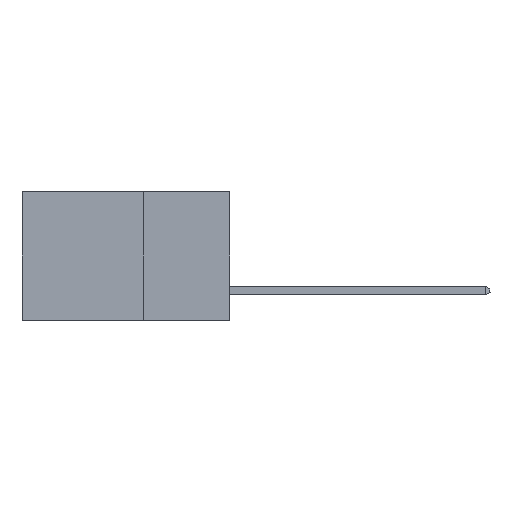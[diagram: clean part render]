
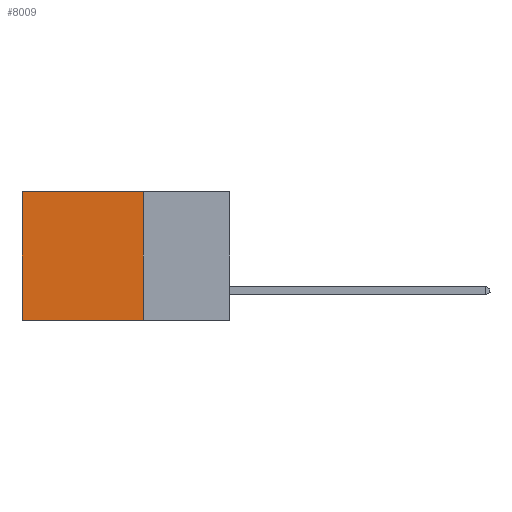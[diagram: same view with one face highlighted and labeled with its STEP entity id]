
A CAD part, left-side view. The second image highlights one B-rep face of the part: STEP entity #8009.
In plain terms, the highlighted planar face has unit normal (-1, 0, 0).
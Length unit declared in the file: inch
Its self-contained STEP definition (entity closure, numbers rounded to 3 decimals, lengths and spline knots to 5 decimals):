
#639 = ORIENTED_EDGE ( 'NONE', *, *, #6393, .F. ) ;
#675 = VECTOR ( 'NONE', #2847, 39.37008 ) ;
#786 = VERTEX_POINT ( 'NONE', #4671 ) ;
#917 = LINE ( 'NONE', #1866, #11841 ) ;
#1866 = CARTESIAN_POINT ( 'NONE',  ( 0.298, 0.6, 0. ) ) ;
#2477 = CARTESIAN_POINT ( 'NONE',  ( 0.298, 0.25, 0. ) ) ;
#2490 = VERTEX_POINT ( 'NONE', #2710 ) ;
#2701 = VECTOR ( 'NONE', #12859, 39.37008 ) ;
#2710 = CARTESIAN_POINT ( 'NONE',  ( 0.298, 0.6, -0.37 ) ) ;
#2847 = DIRECTION ( 'NONE',  ( 0., 1., 0. ) ) ;
#4002 = LINE ( 'NONE', #11662, #2701 ) ;
#4671 = CARTESIAN_POINT ( 'NONE',  ( 0.298, 0.25, -0.37 ) ) ;
#4898 = EDGE_CURVE ( 'NONE', #13296, #786, #13934, .T. ) ;
#5202 = EDGE_LOOP ( 'NONE', ( #8186, #639, #5785, #14836 ) ) ;
#5394 = CARTESIAN_POINT ( 'NONE',  ( 0.298, 0.25, 0. ) ) ;
#5785 = ORIENTED_EDGE ( 'NONE', *, *, #4898, .F. ) ;
#6043 = VECTOR ( 'NONE', #9652, 39.37008 ) ;
#6393 = EDGE_CURVE ( 'NONE', #786, #2490, #12641, .T. ) ;
#6570 = CARTESIAN_POINT ( 'NONE',  ( 0.298, 0.6, 0. ) ) ;
#8009 = ADVANCED_FACE ( 'NONE', ( #10760 ), #11492, .F. ) ;
#8186 = ORIENTED_EDGE ( 'NONE', *, *, #8856, .T. ) ;
#8458 = VERTEX_POINT ( 'NONE', #6570 ) ;
#8856 = EDGE_CURVE ( 'NONE', #8458, #2490, #917, .T. ) ;
#9033 = AXIS2_PLACEMENT_3D ( 'NONE', #10405, #13703, #13801 ) ;
#9123 = DIRECTION ( 'NONE',  ( 0., 0., -1. ) ) ;
#9652 = DIRECTION ( 'NONE',  ( 0., 0., -1. ) ) ;
#10405 = CARTESIAN_POINT ( 'NONE',  ( 0.298, 0.25, 0. ) ) ;
#10760 = FACE_OUTER_BOUND ( 'NONE', #5202, .T. ) ;
#11492 = PLANE ( 'NONE',  #9033 ) ;
#11662 = CARTESIAN_POINT ( 'NONE',  ( 0.298, 0.25, 0. ) ) ;
#11841 = VECTOR ( 'NONE', #9123, 39.37008 ) ;
#12641 = LINE ( 'NONE', #13369, #675 ) ;
#12859 = DIRECTION ( 'NONE',  ( 0., 1., 0. ) ) ;
#12888 = EDGE_CURVE ( 'NONE', #13296, #8458, #4002, .T. ) ;
#13296 = VERTEX_POINT ( 'NONE', #5394 ) ;
#13369 = CARTESIAN_POINT ( 'NONE',  ( 0.298, 0.25, -0.37 ) ) ;
#13703 = DIRECTION ( 'NONE',  ( 1., 0., 0. ) ) ;
#13801 = DIRECTION ( 'NONE',  ( 0., 0., -1. ) ) ;
#13934 = LINE ( 'NONE', #2477, #6043 ) ;
#14836 = ORIENTED_EDGE ( 'NONE', *, *, #12888, .T. ) ;
